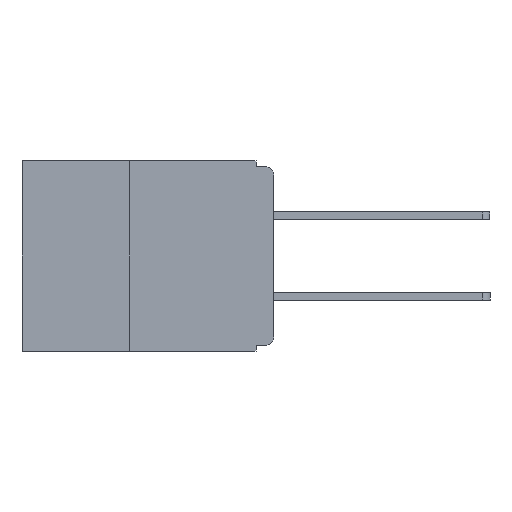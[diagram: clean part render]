
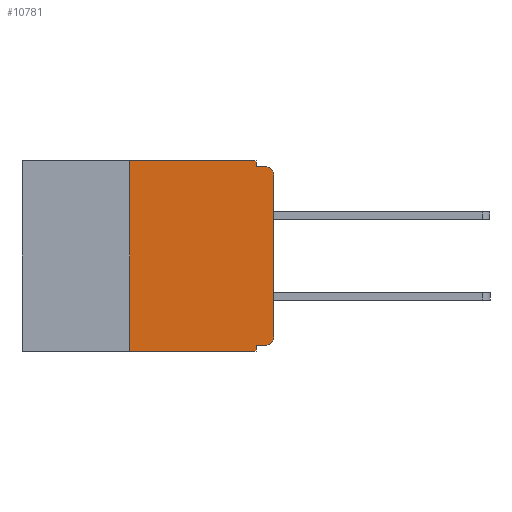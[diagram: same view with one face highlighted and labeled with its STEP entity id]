
A CAD part, left-side view. The second image highlights one B-rep face of the part: STEP entity #10781.
In plain terms, the highlighted planar face has unit normal (-1, 0, 0).
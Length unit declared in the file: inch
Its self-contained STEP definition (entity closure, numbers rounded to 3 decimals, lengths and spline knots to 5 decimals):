
#59 = LINE ( 'NONE', #1898, #11851 ) ;
#234 = DIRECTION ( 'NONE',  ( 0., 0., -1. ) ) ;
#302 = VERTEX_POINT ( 'NONE', #11841 ) ;
#680 = ORIENTED_EDGE ( 'NONE', *, *, #7105, .F. ) ;
#755 = VERTEX_POINT ( 'NONE', #9084 ) ;
#1165 = CARTESIAN_POINT ( 'NONE',  ( 0., 0.25, 0. ) ) ;
#1274 = CARTESIAN_POINT ( 'NONE',  ( 0., 0.25, -0.33 ) ) ;
#1542 = EDGE_CURVE ( 'NONE', #6280, #3994, #11695, .T. ) ;
#1773 = VECTOR ( 'NONE', #12541, 39.37008 ) ;
#1898 = CARTESIAN_POINT ( 'NONE',  ( 0., 0.031, -0.33 ) ) ;
#1943 = CARTESIAN_POINT ( 'NONE',  ( 0., 0.031, 0. ) ) ;
#2214 = EDGE_CURVE ( 'NONE', #13034, #755, #59, .T. ) ;
#2371 = DIRECTION ( 'NONE',  ( -1., 0., 0. ) ) ;
#2388 = DIRECTION ( 'NONE',  ( 0., 0., -1. ) ) ;
#2536 = VECTOR ( 'NONE', #3375, 39.37008 ) ;
#2547 = EDGE_LOOP ( 'NONE', ( #10393, #9343, #11075, #12126, #2658, #13575, #6377, #3157, #680, #7918 ) ) ;
#2576 = DIRECTION ( 'NONE',  ( 0., 0., -1. ) ) ;
#2658 = ORIENTED_EDGE ( 'NONE', *, *, #13272, .F. ) ;
#2685 = VERTEX_POINT ( 'NONE', #1274 ) ;
#2741 = EDGE_CURVE ( 'NONE', #302, #6351, #10827, .T. ) ;
#2894 = LINE ( 'NONE', #11736, #8771 ) ;
#3142 = AXIS2_PLACEMENT_3D ( 'NONE', #6156, #2371, #2388 ) ;
#3157 = ORIENTED_EDGE ( 'NONE', *, *, #2214, .F. ) ;
#3375 = DIRECTION ( 'NONE',  ( 0., 1., 0. ) ) ;
#3495 = DIRECTION ( 'NONE',  ( 0., -1., 0. ) ) ;
#3575 = DIRECTION ( 'NONE',  ( 1., 0., 0. ) ) ;
#3579 = CARTESIAN_POINT ( 'NONE',  ( 0., 0., -0.32 ) ) ;
#3801 = LINE ( 'NONE', #10148, #6727 ) ;
#3835 = VERTEX_POINT ( 'NONE', #5449 ) ;
#3994 = VERTEX_POINT ( 'NONE', #11279 ) ;
#4423 = EDGE_CURVE ( 'NONE', #7233, #3835, #9431, .T. ) ;
#4830 = CARTESIAN_POINT ( 'NONE',  ( 0., 0.25, -0.33 ) ) ;
#4964 = CARTESIAN_POINT ( 'NONE',  ( 0., 0.031, -0.32 ) ) ;
#5119 = DIRECTION ( 'NONE',  ( 0., 0., 1. ) ) ;
#5174 = AXIS2_PLACEMENT_3D ( 'NONE', #9112, #3575, #11310 ) ;
#5280 = DIRECTION ( 'NONE',  ( 0., 0., -1. ) ) ;
#5286 = DIRECTION ( 'NONE',  ( -1., 0., 0. ) ) ;
#5315 = CARTESIAN_POINT ( 'NONE',  ( 0., 0.015, -0.025 ) ) ;
#5443 = LINE ( 'NONE', #3579, #2536 ) ;
#5449 = CARTESIAN_POINT ( 'NONE',  ( 0., 0.031, -0.01 ) ) ;
#5757 = VECTOR ( 'NONE', #234, 39.37008 ) ;
#6156 = CARTESIAN_POINT ( 'NONE',  ( 0., 0.015, -0.305 ) ) ;
#6280 = VERTEX_POINT ( 'NONE', #11218 ) ;
#6351 = VERTEX_POINT ( 'NONE', #10729 ) ;
#6377 = ORIENTED_EDGE ( 'NONE', *, *, #14017, .T. ) ;
#6546 = FACE_OUTER_BOUND ( 'NONE', #2547, .T. ) ;
#6727 = VECTOR ( 'NONE', #3495, 39.37008 ) ;
#7105 = EDGE_CURVE ( 'NONE', #6280, #13034, #5443, .T. ) ;
#7233 = VERTEX_POINT ( 'NONE', #1943 ) ;
#7631 = DIRECTION ( 'NONE',  ( 0., -1., 0. ) ) ;
#7918 = ORIENTED_EDGE ( 'NONE', *, *, #1542, .T. ) ;
#8771 = VECTOR ( 'NONE', #5119, 39.37008 ) ;
#9084 = CARTESIAN_POINT ( 'NONE',  ( 0., 0.031, -0.33 ) ) ;
#9112 = CARTESIAN_POINT ( 'NONE',  ( 0., 0.437, 0. ) ) ;
#9343 = ORIENTED_EDGE ( 'NONE', *, *, #2741, .T. ) ;
#9363 = CARTESIAN_POINT ( 'NONE',  ( 0., 0., -0.01 ) ) ;
#9431 = LINE ( 'NONE', #11664, #5757 ) ;
#9846 = VECTOR ( 'NONE', #12638, 39.37008 ) ;
#9851 = CARTESIAN_POINT ( 'NONE',  ( 0., 0.437, 0. ) ) ;
#10148 = CARTESIAN_POINT ( 'NONE',  ( 0., 0.437, -0.33 ) ) ;
#10215 = PLANE ( 'NONE',  #5174 ) ;
#10249 = LINE ( 'NONE', #4830, #1773 ) ;
#10393 = ORIENTED_EDGE ( 'NONE', *, *, #12176, .T. ) ;
#10642 = VERTEX_POINT ( 'NONE', #1165 ) ;
#10729 = CARTESIAN_POINT ( 'NONE',  ( 0., 0.015, -0.01 ) ) ;
#10781 = ADVANCED_FACE ( 'NONE', ( #6546 ), #10215, .F. ) ;
#10827 = CIRCLE ( 'NONE', #10939, 0.015 ) ;
#10939 = AXIS2_PLACEMENT_3D ( 'NONE', #5315, #5286, #5280 ) ;
#11075 = ORIENTED_EDGE ( 'NONE', *, *, #12086, .F. ) ;
#11218 = CARTESIAN_POINT ( 'NONE',  ( 0., 0.015, -0.32 ) ) ;
#11279 = CARTESIAN_POINT ( 'NONE',  ( 0., 0., -0.305 ) ) ;
#11310 = DIRECTION ( 'NONE',  ( 0., 0., -1. ) ) ;
#11664 = CARTESIAN_POINT ( 'NONE',  ( 0., 0.031, 0. ) ) ;
#11695 = CIRCLE ( 'NONE', #3142, 0.015 ) ;
#11736 = CARTESIAN_POINT ( 'NONE',  ( 0., 0., 0. ) ) ;
#11841 = CARTESIAN_POINT ( 'NONE',  ( 0., 0., -0.025 ) ) ;
#11851 = VECTOR ( 'NONE', #2576, 39.37008 ) ;
#12086 = EDGE_CURVE ( 'NONE', #3835, #6351, #13022, .T. ) ;
#12126 = ORIENTED_EDGE ( 'NONE', *, *, #4423, .F. ) ;
#12176 = EDGE_CURVE ( 'NONE', #3994, #302, #2894, .T. ) ;
#12541 = DIRECTION ( 'NONE',  ( 0., 0., 1. ) ) ;
#12638 = DIRECTION ( 'NONE',  ( 0., -1., 0. ) ) ;
#12938 = EDGE_CURVE ( 'NONE', #2685, #10642, #10249, .T. ) ;
#13022 = LINE ( 'NONE', #9363, #9846 ) ;
#13034 = VERTEX_POINT ( 'NONE', #4964 ) ;
#13272 = EDGE_CURVE ( 'NONE', #10642, #7233, #14054, .T. ) ;
#13575 = ORIENTED_EDGE ( 'NONE', *, *, #12938, .F. ) ;
#13731 = VECTOR ( 'NONE', #7631, 39.37008 ) ;
#14017 = EDGE_CURVE ( 'NONE', #2685, #755, #3801, .T. ) ;
#14054 = LINE ( 'NONE', #9851, #13731 ) ;
